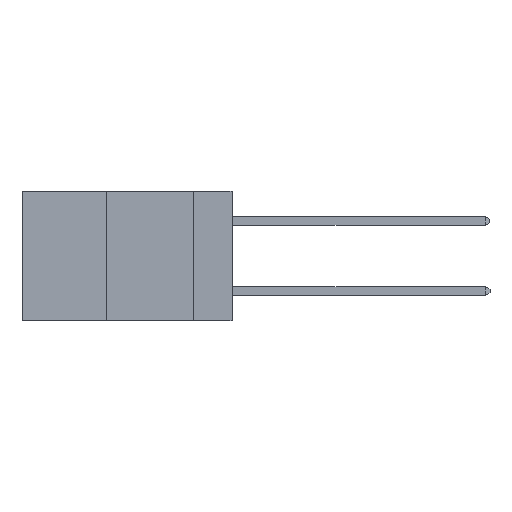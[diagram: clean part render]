
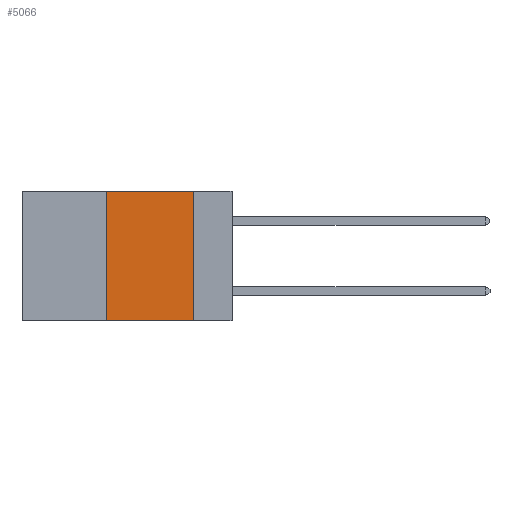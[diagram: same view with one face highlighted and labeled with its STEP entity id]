
A CAD part, left-side view. The second image highlights one B-rep face of the part: STEP entity #5066.
In plain terms, the highlighted planar face has unit normal (-1, 0, 0).
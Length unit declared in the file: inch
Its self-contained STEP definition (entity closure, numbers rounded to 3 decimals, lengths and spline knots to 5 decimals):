
#107 = ORIENTED_EDGE ( 'NONE', *, *, #9225, .F. ) ;
#805 = AXIS2_PLACEMENT_3D ( 'NONE', #9275, #12147, #6357 ) ;
#885 = DIRECTION ( 'NONE',  ( 0., 0., 1. ) ) ;
#1151 = VERTEX_POINT ( 'NONE', #6265 ) ;
#1325 = PLANE ( 'NONE',  #805 ) ;
#2105 = CARTESIAN_POINT ( 'NONE',  ( 0., 0.11, 0. ) ) ;
#2149 = VECTOR ( 'NONE', #4893, 39.37008 ) ;
#3790 = CARTESIAN_POINT ( 'NONE',  ( 0., 0.11, 0. ) ) ;
#4013 = ORIENTED_EDGE ( 'NONE', *, *, #10908, .F. ) ;
#4036 = VECTOR ( 'NONE', #885, 39.37008 ) ;
#4685 = VECTOR ( 'NONE', #6106, 39.37008 ) ;
#4893 = DIRECTION ( 'NONE',  ( 0., -1., 0. ) ) ;
#4951 = VECTOR ( 'NONE', #7420, 39.37008 ) ;
#5066 = ADVANCED_FACE ( 'NONE', ( #10855 ), #1325, .F. ) ;
#5248 = LINE ( 'NONE', #12212, #4951 ) ;
#5999 = VERTEX_POINT ( 'NONE', #7934 ) ;
#6106 = DIRECTION ( 'NONE',  ( 0., 0., -1. ) ) ;
#6265 = CARTESIAN_POINT ( 'NONE',  ( 0., 0.36, -0.37 ) ) ;
#6357 = DIRECTION ( 'NONE',  ( 0., 0., -1. ) ) ;
#7271 = LINE ( 'NONE', #12659, #4036 ) ;
#7280 = LINE ( 'NONE', #2105, #4685 ) ;
#7420 = DIRECTION ( 'NONE',  ( 0., -1., 0. ) ) ;
#7934 = CARTESIAN_POINT ( 'NONE',  ( 0., 0.11, -0.37 ) ) ;
#8976 = EDGE_CURVE ( 'NONE', #1151, #5999, #9731, .T. ) ;
#9225 = EDGE_CURVE ( 'NONE', #9710, #5999, #7280, .T. ) ;
#9275 = CARTESIAN_POINT ( 'NONE',  ( 0., 0.6, 0. ) ) ;
#9710 = VERTEX_POINT ( 'NONE', #3790 ) ;
#9731 = LINE ( 'NONE', #11662, #2149 ) ;
#10418 = ORIENTED_EDGE ( 'NONE', *, *, #8976, .T. ) ;
#10534 = EDGE_CURVE ( 'NONE', #1151, #10762, #7271, .T. ) ;
#10762 = VERTEX_POINT ( 'NONE', #12002 ) ;
#10855 = FACE_OUTER_BOUND ( 'NONE', #11890, .T. ) ;
#10908 = EDGE_CURVE ( 'NONE', #10762, #9710, #5248, .T. ) ;
#11662 = CARTESIAN_POINT ( 'NONE',  ( 0., 0.6, -0.37 ) ) ;
#11786 = ORIENTED_EDGE ( 'NONE', *, *, #10534, .F. ) ;
#11890 = EDGE_LOOP ( 'NONE', ( #107, #4013, #11786, #10418 ) ) ;
#12002 = CARTESIAN_POINT ( 'NONE',  ( 0., 0.36, 0. ) ) ;
#12147 = DIRECTION ( 'NONE',  ( 1., 0., 0. ) ) ;
#12212 = CARTESIAN_POINT ( 'NONE',  ( 0., 0.6, 0. ) ) ;
#12659 = CARTESIAN_POINT ( 'NONE',  ( 0., 0.36, 0. ) ) ;
